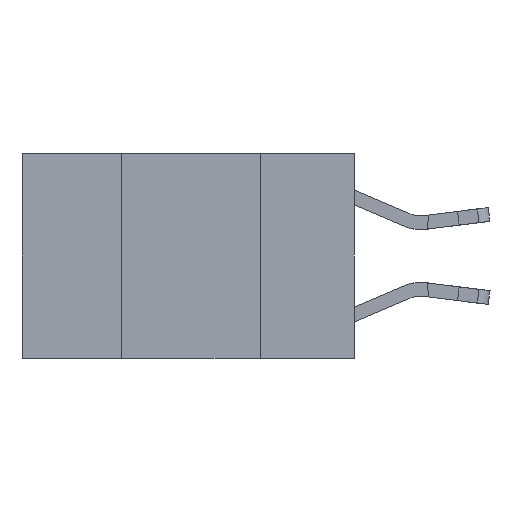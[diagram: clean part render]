
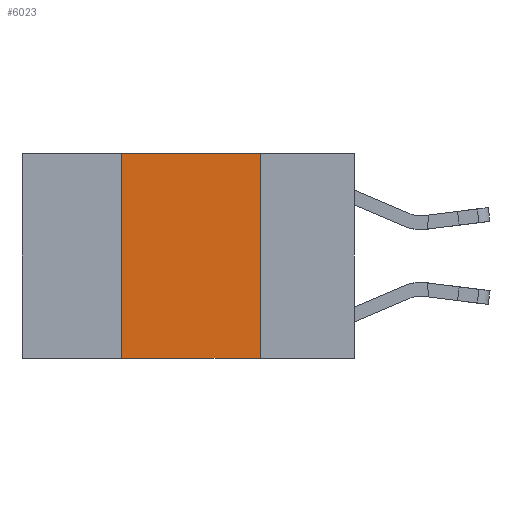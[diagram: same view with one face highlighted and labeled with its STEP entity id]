
A CAD part, left-side view. The second image highlights one B-rep face of the part: STEP entity #6023.
In plain terms, the highlighted planar face has unit normal (-1, 0, 0).
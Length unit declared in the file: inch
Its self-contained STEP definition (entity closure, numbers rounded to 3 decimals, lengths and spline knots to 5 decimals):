
#314 = DIRECTION ( 'NONE',  ( 0., 0., 1. ) ) ;
#599 = LINE ( 'NONE', #16753, #14300 ) ;
#2238 = DIRECTION ( 'NONE',  ( 0., -1., 0. ) ) ;
#2242 = DIRECTION ( 'NONE',  ( 0., -1., 0. ) ) ;
#3438 = VECTOR ( 'NONE', #2242, 39.37008 ) ;
#3966 = LINE ( 'NONE', #9610, #10173 ) ;
#4524 = CARTESIAN_POINT ( 'NONE',  ( 0., 0.42, -0.37 ) ) ;
#4981 = ORIENTED_EDGE ( 'NONE', *, *, #15807, .F. ) ;
#5828 = ORIENTED_EDGE ( 'NONE', *, *, #15887, .F. ) ;
#6023 = ADVANCED_FACE ( 'NONE', ( #9413 ), #11470, .F. ) ;
#6026 = DIRECTION ( 'NONE',  ( 0., 0., -1. ) ) ;
#6226 = VERTEX_POINT ( 'NONE', #15815 ) ;
#6247 = DIRECTION ( 'NONE',  ( 0., 0., -1. ) ) ;
#7103 = EDGE_LOOP ( 'NONE', ( #4981, #5828, #9333, #13267 ) ) ;
#7723 = VERTEX_POINT ( 'NONE', #4524 ) ;
#8283 = EDGE_CURVE ( 'NONE', #7723, #6226, #3966, .T. ) ;
#8925 = LINE ( 'NONE', #10001, #15535 ) ;
#9333 = ORIENTED_EDGE ( 'NONE', *, *, #8283, .F. ) ;
#9413 = FACE_OUTER_BOUND ( 'NONE', #7103, .T. ) ;
#9610 = CARTESIAN_POINT ( 'NONE',  ( 0., 0.42, 0. ) ) ;
#10001 = CARTESIAN_POINT ( 'NONE',  ( 0., 0.17, 0. ) ) ;
#10173 = VECTOR ( 'NONE', #314, 39.37008 ) ;
#10286 = VERTEX_POINT ( 'NONE', #15161 ) ;
#10882 = VERTEX_POINT ( 'NONE', #13818 ) ;
#11470 = PLANE ( 'NONE',  #16283 ) ;
#11486 = CARTESIAN_POINT ( 'NONE',  ( 0., 0.6, -0.37 ) ) ;
#12815 = CARTESIAN_POINT ( 'NONE',  ( 0., 0.6, 0. ) ) ;
#13267 = ORIENTED_EDGE ( 'NONE', *, *, #13812, .T. ) ;
#13812 = EDGE_CURVE ( 'NONE', #7723, #10286, #16679, .T. ) ;
#13818 = CARTESIAN_POINT ( 'NONE',  ( 0., 0.17, 0. ) ) ;
#14151 = DIRECTION ( 'NONE',  ( 1., 0., 0. ) ) ;
#14300 = VECTOR ( 'NONE', #2238, 39.37008 ) ;
#15161 = CARTESIAN_POINT ( 'NONE',  ( 0., 0.17, -0.37 ) ) ;
#15535 = VECTOR ( 'NONE', #6026, 39.37008 ) ;
#15807 = EDGE_CURVE ( 'NONE', #10882, #10286, #8925, .T. ) ;
#15815 = CARTESIAN_POINT ( 'NONE',  ( 0., 0.42, 0. ) ) ;
#15887 = EDGE_CURVE ( 'NONE', #6226, #10882, #599, .T. ) ;
#16283 = AXIS2_PLACEMENT_3D ( 'NONE', #12815, #14151, #6247 ) ;
#16679 = LINE ( 'NONE', #11486, #3438 ) ;
#16753 = CARTESIAN_POINT ( 'NONE',  ( 0., 0.6, 0. ) ) ;
